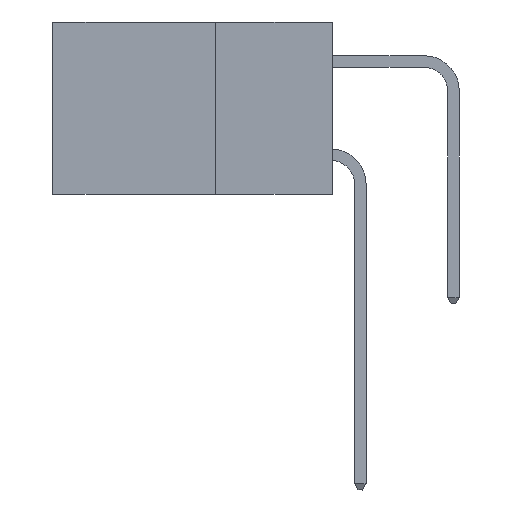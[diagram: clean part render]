
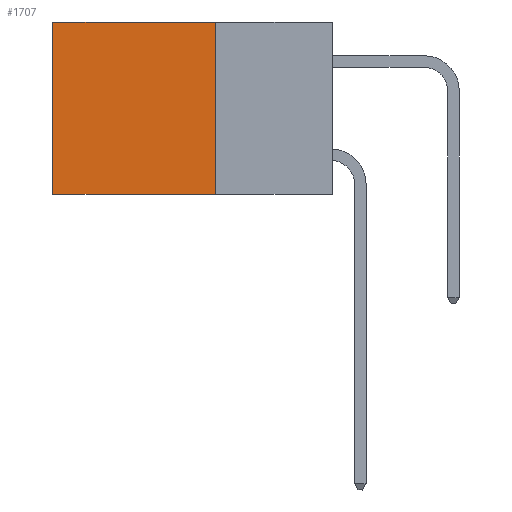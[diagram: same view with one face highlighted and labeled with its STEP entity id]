
A CAD part, left-side view. The second image highlights one B-rep face of the part: STEP entity #1707.
In plain terms, the highlighted planar face has unit normal (-1, 0, 0).
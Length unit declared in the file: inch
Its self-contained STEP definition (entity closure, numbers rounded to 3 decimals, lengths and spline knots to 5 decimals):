
#938 = DIRECTION ( 'NONE',  ( 0., 0., -1. ) ) ;
#1320 = DIRECTION ( 'NONE',  ( 1., 0., 0. ) ) ;
#1707 = ADVANCED_FACE ( 'NONE', ( #8793 ), #2721, .F. ) ;
#2110 = CARTESIAN_POINT ( 'NONE',  ( 0.298, 0.25, 0. ) ) ;
#2139 = VECTOR ( 'NONE', #11070, 39.37008 ) ;
#2151 = VERTEX_POINT ( 'NONE', #12138 ) ;
#2204 = VECTOR ( 'NONE', #9416, 39.37008 ) ;
#2721 = PLANE ( 'NONE',  #9493 ) ;
#2742 = VERTEX_POINT ( 'NONE', #10655 ) ;
#4513 = CARTESIAN_POINT ( 'NONE',  ( 0.298, 0.25, 0. ) ) ;
#4515 = VERTEX_POINT ( 'NONE', #4513 ) ;
#5621 = EDGE_CURVE ( 'NONE', #4515, #2151, #11354, .T. ) ;
#6096 = LINE ( 'NONE', #8940, #8687 ) ;
#6121 = EDGE_LOOP ( 'NONE', ( #13262, #8369, #12652, #8881 ) ) ;
#6729 = EDGE_CURVE ( 'NONE', #2742, #8113, #6096, .T. ) ;
#6820 = EDGE_CURVE ( 'NONE', #2151, #8113, #13214, .T. ) ;
#7254 = CARTESIAN_POINT ( 'NONE',  ( 0.298, 0.25, 0. ) ) ;
#8113 = VERTEX_POINT ( 'NONE', #11167 ) ;
#8331 = VECTOR ( 'NONE', #12209, 39.37008 ) ;
#8369 = ORIENTED_EDGE ( 'NONE', *, *, #6820, .F. ) ;
#8687 = VECTOR ( 'NONE', #10015, 39.37008 ) ;
#8793 = FACE_OUTER_BOUND ( 'NONE', #6121, .T. ) ;
#8881 = ORIENTED_EDGE ( 'NONE', *, *, #9278, .T. ) ;
#8940 = CARTESIAN_POINT ( 'NONE',  ( 0.298, 0.6, 0. ) ) ;
#9278 = EDGE_CURVE ( 'NONE', #4515, #2742, #11089, .T. ) ;
#9416 = DIRECTION ( 'NONE',  ( 0., 1., 0. ) ) ;
#9493 = AXIS2_PLACEMENT_3D ( 'NONE', #10296, #1320, #938 ) ;
#10015 = DIRECTION ( 'NONE',  ( 0., 0., -1. ) ) ;
#10296 = CARTESIAN_POINT ( 'NONE',  ( 0.298, 0.25, 0. ) ) ;
#10655 = CARTESIAN_POINT ( 'NONE',  ( 0.298, 0.6, 0. ) ) ;
#11070 = DIRECTION ( 'NONE',  ( 0., 0., -1. ) ) ;
#11089 = LINE ( 'NONE', #7254, #2204 ) ;
#11167 = CARTESIAN_POINT ( 'NONE',  ( 0.298, 0.6, -0.37 ) ) ;
#11354 = LINE ( 'NONE', #2110, #2139 ) ;
#12138 = CARTESIAN_POINT ( 'NONE',  ( 0.298, 0.25, -0.37 ) ) ;
#12209 = DIRECTION ( 'NONE',  ( 0., 1., 0. ) ) ;
#12652 = ORIENTED_EDGE ( 'NONE', *, *, #5621, .F. ) ;
#13214 = LINE ( 'NONE', #14248, #8331 ) ;
#13262 = ORIENTED_EDGE ( 'NONE', *, *, #6729, .T. ) ;
#14248 = CARTESIAN_POINT ( 'NONE',  ( 0.298, 0.25, -0.37 ) ) ;
